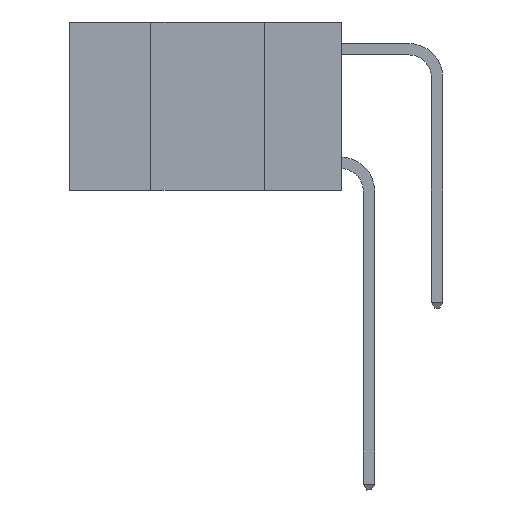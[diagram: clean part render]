
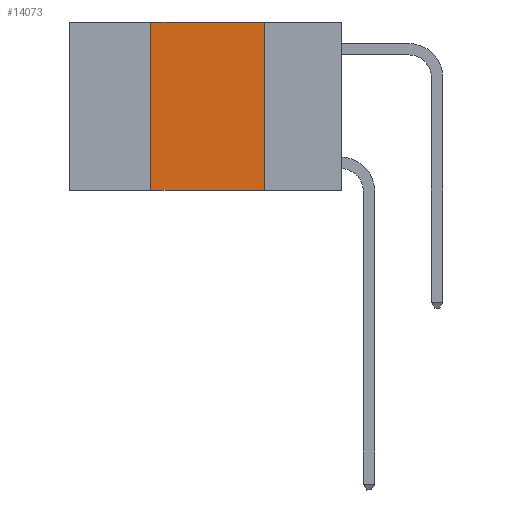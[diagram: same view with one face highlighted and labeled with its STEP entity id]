
A CAD part, left-side view. The second image highlights one B-rep face of the part: STEP entity #14073.
In plain terms, the highlighted planar face has unit normal (-1, 0, 0).
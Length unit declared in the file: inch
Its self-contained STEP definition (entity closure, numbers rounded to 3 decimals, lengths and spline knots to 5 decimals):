
#492 = CARTESIAN_POINT ( 'NONE',  ( 0., 0.6, -0.37 ) ) ;
#807 = CARTESIAN_POINT ( 'NONE',  ( 0., 0.17, -0.37 ) ) ;
#1117 = DIRECTION ( 'NONE',  ( 0., 0., -1. ) ) ;
#1347 = ORIENTED_EDGE ( 'NONE', *, *, #7065, .F. ) ;
#1376 = ORIENTED_EDGE ( 'NONE', *, *, #12062, .T. ) ;
#1991 = CARTESIAN_POINT ( 'NONE',  ( 0., 0.17, 0. ) ) ;
#2865 = FACE_OUTER_BOUND ( 'NONE', #15170, .T. ) ;
#3390 = EDGE_CURVE ( 'NONE', #7040, #15111, #16268, .T. ) ;
#4174 = VECTOR ( 'NONE', #4451, 39.37008 ) ;
#4411 = DIRECTION ( 'NONE',  ( 0., -1., 0. ) ) ;
#4451 = DIRECTION ( 'NONE',  ( 0., 0., 1. ) ) ;
#5498 = DIRECTION ( 'NONE',  ( 1., 0., 0. ) ) ;
#5751 = VERTEX_POINT ( 'NONE', #807 ) ;
#6356 = DIRECTION ( 'NONE',  ( 0., -1., 0. ) ) ;
#7040 = VERTEX_POINT ( 'NONE', #11750 ) ;
#7065 = EDGE_CURVE ( 'NONE', #12517, #5751, #10445, .T. ) ;
#7203 = AXIS2_PLACEMENT_3D ( 'NONE', #9632, #5498, #9825 ) ;
#7806 = CARTESIAN_POINT ( 'NONE',  ( 0., 0.17, 0. ) ) ;
#7979 = VECTOR ( 'NONE', #6356, 39.37008 ) ;
#8474 = VECTOR ( 'NONE', #1117, 39.37008 ) ;
#9632 = CARTESIAN_POINT ( 'NONE',  ( 0., 0.6, 0. ) ) ;
#9825 = DIRECTION ( 'NONE',  ( 0., 0., -1. ) ) ;
#10445 = LINE ( 'NONE', #7806, #8474 ) ;
#10844 = LINE ( 'NONE', #492, #11097 ) ;
#11097 = VECTOR ( 'NONE', #4411, 39.37008 ) ;
#11373 = ORIENTED_EDGE ( 'NONE', *, *, #3390, .F. ) ;
#11476 = CARTESIAN_POINT ( 'NONE',  ( 0., 0.42, 0. ) ) ;
#11637 = EDGE_CURVE ( 'NONE', #15111, #12517, #13061, .T. ) ;
#11750 = CARTESIAN_POINT ( 'NONE',  ( 0., 0.42, -0.37 ) ) ;
#12062 = EDGE_CURVE ( 'NONE', #7040, #5751, #10844, .T. ) ;
#12517 = VERTEX_POINT ( 'NONE', #1991 ) ;
#13061 = LINE ( 'NONE', #13408, #7979 ) ;
#13408 = CARTESIAN_POINT ( 'NONE',  ( 0., 0.6, 0. ) ) ;
#13705 = PLANE ( 'NONE',  #7203 ) ;
#14073 = ADVANCED_FACE ( 'NONE', ( #2865 ), #13705, .F. ) ;
#15111 = VERTEX_POINT ( 'NONE', #11476 ) ;
#15127 = CARTESIAN_POINT ( 'NONE',  ( 0., 0.42, 0. ) ) ;
#15170 = EDGE_LOOP ( 'NONE', ( #1347, #16989, #11373, #1376 ) ) ;
#16268 = LINE ( 'NONE', #15127, #4174 ) ;
#16989 = ORIENTED_EDGE ( 'NONE', *, *, #11637, .F. ) ;
